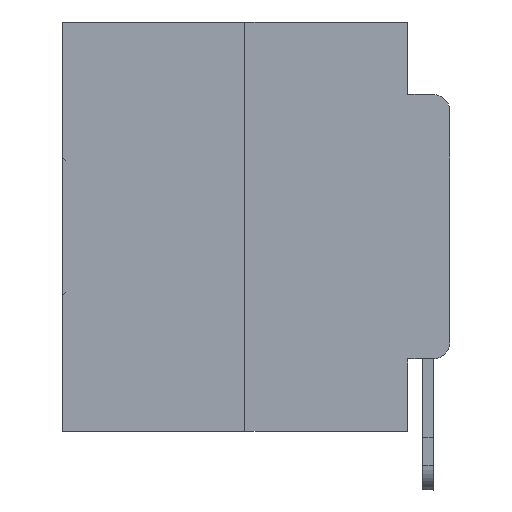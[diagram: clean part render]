
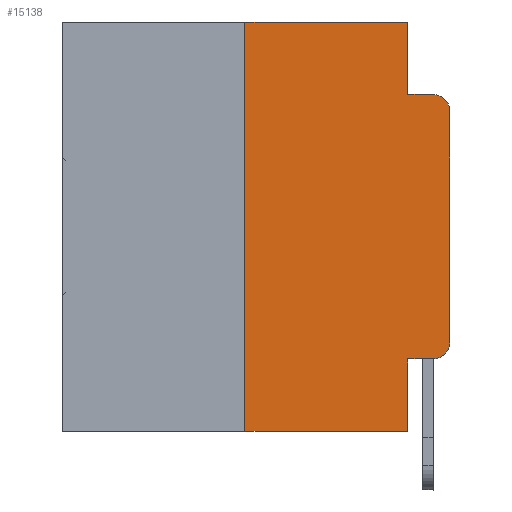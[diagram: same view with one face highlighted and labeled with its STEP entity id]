
A CAD part, left-side view. The second image highlights one B-rep face of the part: STEP entity #15138.
In plain terms, the highlighted planar face has unit normal (-1, 0, 0).
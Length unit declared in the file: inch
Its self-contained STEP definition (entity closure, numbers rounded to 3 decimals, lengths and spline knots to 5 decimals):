
#338 = VERTEX_POINT ( 'NONE', #22180 ) ;
#346 = ORIENTED_EDGE ( 'NONE', *, *, #17309, .T. ) ;
#470 = CARTESIAN_POINT ( 'NONE',  ( 0., 0.473, -0.5 ) ) ;
#932 = ORIENTED_EDGE ( 'NONE', *, *, #24200, .F. ) ;
#1001 = FACE_OUTER_BOUND ( 'NONE', #10277, .T. ) ;
#2216 = VERTEX_POINT ( 'NONE', #2269 ) ;
#2269 = CARTESIAN_POINT ( 'NONE',  ( 0., 0.02, -0.0885 ) ) ;
#2385 = DIRECTION ( 'NONE',  ( 0., -1., 0. ) ) ;
#2701 = CARTESIAN_POINT ( 'NONE',  ( 0., 0.051, -0.4115 ) ) ;
#2968 = ORIENTED_EDGE ( 'NONE', *, *, #15614, .F. ) ;
#3342 = CARTESIAN_POINT ( 'NONE',  ( 0., 0.051, 0. ) ) ;
#3346 = DIRECTION ( 'NONE',  ( -1., 0., 0. ) ) ;
#3435 = DIRECTION ( 'NONE',  ( 0., 0., -1. ) ) ;
#3472 = CARTESIAN_POINT ( 'NONE',  ( 0., 0.02, -0.4115 ) ) ;
#4378 = EDGE_CURVE ( 'NONE', #18401, #18158, #7687, .T. ) ;
#4422 = CARTESIAN_POINT ( 'NONE',  ( 0., 0.051, -0.5 ) ) ;
#4756 = VECTOR ( 'NONE', #2385, 39.37008 ) ;
#5483 = LINE ( 'NONE', #3342, #16005 ) ;
#5917 = CARTESIAN_POINT ( 'NONE',  ( 0., 0., -0.1085 ) ) ;
#5981 = CARTESIAN_POINT ( 'NONE',  ( 0., 0.02, -0.3915 ) ) ;
#6166 = AXIS2_PLACEMENT_3D ( 'NONE', #5981, #15501, #29954 ) ;
#6793 = CARTESIAN_POINT ( 'NONE',  ( 0., 0., -0.3915 ) ) ;
#7687 = LINE ( 'NONE', #28348, #8428 ) ;
#8052 = VECTOR ( 'NONE', #19342, 39.37008 ) ;
#8428 = VECTOR ( 'NONE', #14125, 39.37008 ) ;
#8809 = DIRECTION ( 'NONE',  ( 0., -1., 0. ) ) ;
#9569 = CARTESIAN_POINT ( 'NONE',  ( 0., 0.25, 0. ) ) ;
#9672 = VECTOR ( 'NONE', #21580, 39.37008 ) ;
#10228 = ORIENTED_EDGE ( 'NONE', *, *, #4378, .F. ) ;
#10277 = EDGE_LOOP ( 'NONE', ( #14293, #17628, #21821, #2968, #932, #28139, #21145, #10228, #17350, #346 ) ) ;
#11912 = DIRECTION ( 'NONE',  ( 0., 0., -1. ) ) ;
#11953 = AXIS2_PLACEMENT_3D ( 'NONE', #18954, #13899, #11912 ) ;
#12637 = VERTEX_POINT ( 'NONE', #3472 ) ;
#13619 = CARTESIAN_POINT ( 'NONE',  ( 0., 0.051, -0.4115 ) ) ;
#13899 = DIRECTION ( 'NONE',  ( 1., 0., 0. ) ) ;
#14125 = DIRECTION ( 'NONE',  ( 0., 0., -1. ) ) ;
#14293 = ORIENTED_EDGE ( 'NONE', *, *, #15130, .T. ) ;
#14340 = CARTESIAN_POINT ( 'NONE',  ( 0., 0.473, 0. ) ) ;
#14908 = CIRCLE ( 'NONE', #24512, 0.02 ) ;
#15129 = VERTEX_POINT ( 'NONE', #6793 ) ;
#15130 = EDGE_CURVE ( 'NONE', #15129, #23067, #15305, .T. ) ;
#15138 = ADVANCED_FACE ( 'NONE', ( #1001 ), #28214, .F. ) ;
#15305 = LINE ( 'NONE', #25848, #20943 ) ;
#15501 = DIRECTION ( 'NONE',  ( -1., 0., 0. ) ) ;
#15614 = EDGE_CURVE ( 'NONE', #338, #22535, #5483, .T. ) ;
#16005 = VECTOR ( 'NONE', #3435, 39.37008 ) ;
#16571 = EDGE_CURVE ( 'NONE', #17777, #19351, #20050, .T. ) ;
#17261 = CARTESIAN_POINT ( 'NONE',  ( 0., 0.02, -0.1085 ) ) ;
#17309 = EDGE_CURVE ( 'NONE', #12637, #15129, #30125, .T. ) ;
#17350 = ORIENTED_EDGE ( 'NONE', *, *, #23927, .T. ) ;
#17628 = ORIENTED_EDGE ( 'NONE', *, *, #31024, .T. ) ;
#17777 = VERTEX_POINT ( 'NONE', #22271 ) ;
#18158 = VERTEX_POINT ( 'NONE', #4422 ) ;
#18401 = VERTEX_POINT ( 'NONE', #2701 ) ;
#18714 = LINE ( 'NONE', #470, #4756 ) ;
#18954 = CARTESIAN_POINT ( 'NONE',  ( 0., 0.473, 0. ) ) ;
#19056 = DIRECTION ( 'NONE',  ( 0., 0., 1. ) ) ;
#19342 = DIRECTION ( 'NONE',  ( 0., 0., 1. ) ) ;
#19351 = VERTEX_POINT ( 'NONE', #23523 ) ;
#20050 = LINE ( 'NONE', #9569, #8052 ) ;
#20943 = VECTOR ( 'NONE', #19056, 39.37008 ) ;
#21145 = ORIENTED_EDGE ( 'NONE', *, *, #31110, .T. ) ;
#21147 = DIRECTION ( 'NONE',  ( 0., 0., -1. ) ) ;
#21340 = VECTOR ( 'NONE', #8809, 39.37008 ) ;
#21427 = LINE ( 'NONE', #25544, #30792 ) ;
#21580 = DIRECTION ( 'NONE',  ( 0., -1., 0. ) ) ;
#21821 = ORIENTED_EDGE ( 'NONE', *, *, #30247, .F. ) ;
#22061 = LINE ( 'NONE', #14340, #9672 ) ;
#22180 = CARTESIAN_POINT ( 'NONE',  ( 0., 0.051, 0. ) ) ;
#22271 = CARTESIAN_POINT ( 'NONE',  ( 0., 0.25, -0.5 ) ) ;
#22535 = VERTEX_POINT ( 'NONE', #27385 ) ;
#23067 = VERTEX_POINT ( 'NONE', #5917 ) ;
#23523 = CARTESIAN_POINT ( 'NONE',  ( 0., 0.25, 0. ) ) ;
#23927 = EDGE_CURVE ( 'NONE', #18401, #12637, #28030, .T. ) ;
#24200 = EDGE_CURVE ( 'NONE', #19351, #338, #22061, .T. ) ;
#24512 = AXIS2_PLACEMENT_3D ( 'NONE', #17261, #3346, #21147 ) ;
#25544 = CARTESIAN_POINT ( 'NONE',  ( 0., 0.051, -0.0885 ) ) ;
#25848 = CARTESIAN_POINT ( 'NONE',  ( 0., 0., 0. ) ) ;
#25856 = DIRECTION ( 'NONE',  ( 0., -1., 0. ) ) ;
#27385 = CARTESIAN_POINT ( 'NONE',  ( 0., 0.051, -0.0885 ) ) ;
#28030 = LINE ( 'NONE', #13619, #21340 ) ;
#28139 = ORIENTED_EDGE ( 'NONE', *, *, #16571, .F. ) ;
#28214 = PLANE ( 'NONE',  #11953 ) ;
#28348 = CARTESIAN_POINT ( 'NONE',  ( 0., 0.051, 0. ) ) ;
#29954 = DIRECTION ( 'NONE',  ( 0., 0., -1. ) ) ;
#30125 = CIRCLE ( 'NONE', #6166, 0.02 ) ;
#30247 = EDGE_CURVE ( 'NONE', #22535, #2216, #21427, .T. ) ;
#30792 = VECTOR ( 'NONE', #25856, 39.37008 ) ;
#31024 = EDGE_CURVE ( 'NONE', #23067, #2216, #14908, .T. ) ;
#31110 = EDGE_CURVE ( 'NONE', #17777, #18158, #18714, .T. ) ;
